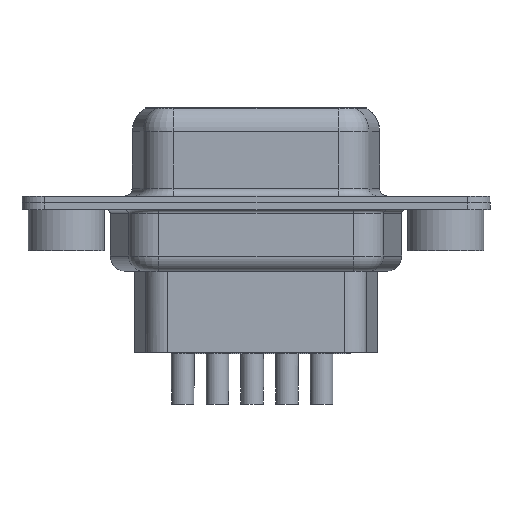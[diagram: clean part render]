
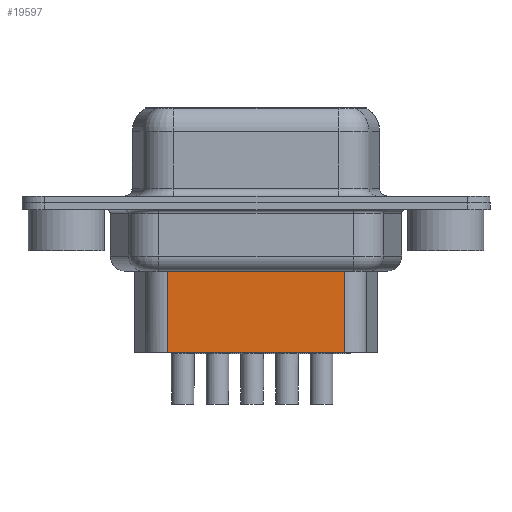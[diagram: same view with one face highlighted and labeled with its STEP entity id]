
A CAD part, front view. The second image highlights one B-rep face of the part: STEP entity #19597.
In plain terms, the highlighted planar face has unit normal (0, -1, 0).
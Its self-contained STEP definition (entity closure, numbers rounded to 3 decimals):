
#93 = VECTOR ( 'NONE', #19557, 1000. ) ;
#923 = VECTOR ( 'NONE', #13275, 1000. ) ;
#1886 = ORIENTED_EDGE ( 'NONE', *, *, #13382, .T. ) ;
#2346 = CARTESIAN_POINT ( 'NONE',  ( 6.701, -3.5, -9.85 ) ) ;
#2972 = FACE_OUTER_BOUND ( 'NONE', #17703, .T. ) ;
#5528 = VERTEX_POINT ( 'NONE', #19382 ) ;
#7535 = CARTESIAN_POINT ( 'NONE',  ( 6.701, -3.5, -9.85 ) ) ;
#7571 = DIRECTION ( 'NONE',  ( 1., 0., 0. ) ) ;
#7835 = EDGE_CURVE ( 'NONE', #5528, #16566, #17577, .T. ) ;
#9081 = DIRECTION ( 'NONE',  ( -1., 0., 0. ) ) ;
#9852 = CARTESIAN_POINT ( 'NONE',  ( 18.289, -3.5, -9.85 ) ) ;
#10644 = VECTOR ( 'NONE', #9081, 1000. ) ;
#10904 = ORIENTED_EDGE ( 'NONE', *, *, #7835, .F. ) ;
#12308 = ORIENTED_EDGE ( 'NONE', *, *, #21619, .T. ) ;
#12408 = VERTEX_POINT ( 'NONE', #2346 ) ;
#12487 = VECTOR ( 'NONE', #14386, 1000. ) ;
#12737 = CARTESIAN_POINT ( 'NONE',  ( 6.701, -3.5, -3.1 ) ) ;
#12913 = CARTESIAN_POINT ( 'NONE',  ( 6.454, -3.5, -4.097 ) ) ;
#13275 = DIRECTION ( 'NONE',  ( -1., 0., 0. ) ) ;
#13287 = VERTEX_POINT ( 'NONE', #17212 ) ;
#13382 = EDGE_CURVE ( 'NONE', #13287, #12408, #14731, .T. ) ;
#13807 = AXIS2_PLACEMENT_3D ( 'NONE', #12737, #18984, #7571 ) ;
#14386 = DIRECTION ( 'NONE',  ( 0., 0., -1. ) ) ;
#14731 = LINE ( 'NONE', #21357, #93 ) ;
#15133 = LINE ( 'NONE', #12913, #10644 ) ;
#16130 = LINE ( 'NONE', #7535, #923 ) ;
#16566 = VERTEX_POINT ( 'NONE', #9852 ) ;
#17078 = PLANE ( 'NONE',  #13807 ) ;
#17212 = CARTESIAN_POINT ( 'NONE',  ( 6.701, -3.5, -4.097 ) ) ;
#17577 = LINE ( 'NONE', #20066, #12487 ) ;
#17703 = EDGE_LOOP ( 'NONE', ( #10904, #12308, #1886, #21459 ) ) ;
#18709 = EDGE_CURVE ( 'NONE', #16566, #12408, #16130, .T. ) ;
#18984 = DIRECTION ( 'NONE',  ( 0., -1., 0. ) ) ;
#19382 = CARTESIAN_POINT ( 'NONE',  ( 18.289, -3.5, -4.097 ) ) ;
#19557 = DIRECTION ( 'NONE',  ( 0., 0., -1. ) ) ;
#19597 = ADVANCED_FACE ( 'NONE', ( #2972 ), #17078, .T. ) ;
#20066 = CARTESIAN_POINT ( 'NONE',  ( 18.289, -3.5, -3.1 ) ) ;
#21357 = CARTESIAN_POINT ( 'NONE',  ( 6.701, -3.5, -3.1 ) ) ;
#21459 = ORIENTED_EDGE ( 'NONE', *, *, #18709, .F. ) ;
#21619 = EDGE_CURVE ( 'NONE', #5528, #13287, #15133, .T. ) ;
